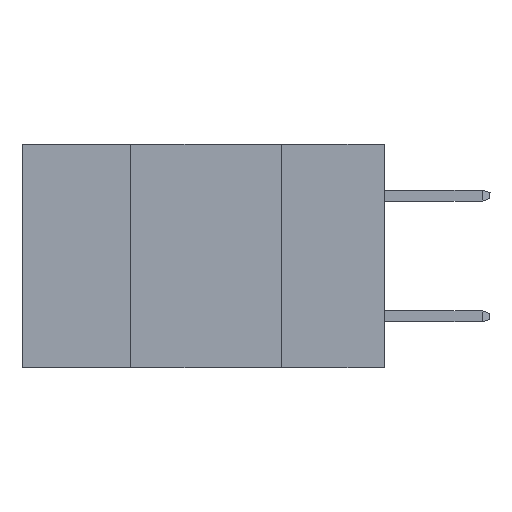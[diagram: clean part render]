
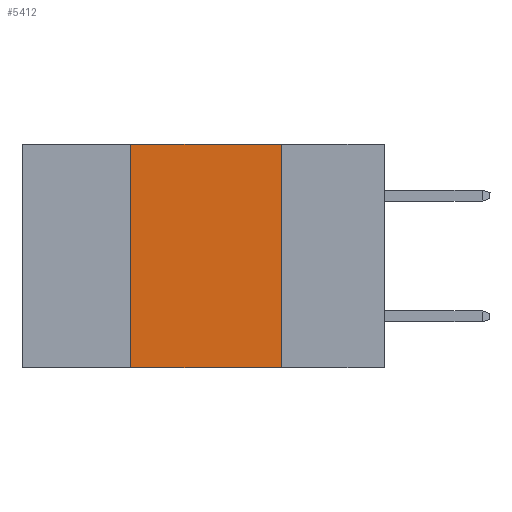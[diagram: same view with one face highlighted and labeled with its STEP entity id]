
A CAD part, left-side view. The second image highlights one B-rep face of the part: STEP entity #5412.
In plain terms, the highlighted planar face has unit normal (-1, 0, 0).
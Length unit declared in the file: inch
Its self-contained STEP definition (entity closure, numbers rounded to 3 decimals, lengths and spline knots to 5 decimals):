
#109 = PLANE ( 'NONE',  #27972 ) ;
#1936 = ORIENTED_EDGE ( 'NONE', *, *, #29631, .T. ) ;
#2480 = CARTESIAN_POINT ( 'NONE',  ( 0., 0.17, -0.37 ) ) ;
#3816 = EDGE_CURVE ( 'NONE', #24427, #20865, #25694, .T. ) ;
#4234 = VECTOR ( 'NONE', #25283, 39.37008 ) ;
#5412 = ADVANCED_FACE ( 'NONE', ( #25995 ), #109, .F. ) ;
#5451 = EDGE_LOOP ( 'NONE', ( #12696, #32093, #16387, #1936 ) ) ;
#5669 = CARTESIAN_POINT ( 'NONE',  ( 0., 0.6, 0. ) ) ;
#8476 = DIRECTION ( 'NONE',  ( 0., 0., -1. ) ) ;
#12034 = DIRECTION ( 'NONE',  ( 0., -1., 0. ) ) ;
#12310 = VECTOR ( 'NONE', #12034, 39.37008 ) ;
#12696 = ORIENTED_EDGE ( 'NONE', *, *, #13010, .F. ) ;
#13010 = EDGE_CURVE ( 'NONE', #31207, #27157, #28992, .T. ) ;
#13232 = CARTESIAN_POINT ( 'NONE',  ( 0., 0.17, 0. ) ) ;
#13496 = CARTESIAN_POINT ( 'NONE',  ( 0., 0.42, -0.37 ) ) ;
#15550 = CARTESIAN_POINT ( 'NONE',  ( 0., 0.6, -0.37 ) ) ;
#16387 = ORIENTED_EDGE ( 'NONE', *, *, #3816, .F. ) ;
#16401 = LINE ( 'NONE', #15550, #29676 ) ;
#18227 = CARTESIAN_POINT ( 'NONE',  ( 0., 0.42, 0. ) ) ;
#20865 = VERTEX_POINT ( 'NONE', #23949 ) ;
#21957 = VECTOR ( 'NONE', #29083, 39.37008 ) ;
#23949 = CARTESIAN_POINT ( 'NONE',  ( 0., 0.42, 0. ) ) ;
#24427 = VERTEX_POINT ( 'NONE', #13496 ) ;
#24458 = DIRECTION ( 'NONE',  ( 1., 0., 0. ) ) ;
#25283 = DIRECTION ( 'NONE',  ( 0., 0., 1. ) ) ;
#25407 = EDGE_CURVE ( 'NONE', #20865, #31207, #32517, .T. ) ;
#25694 = LINE ( 'NONE', #18227, #4234 ) ;
#25995 = FACE_OUTER_BOUND ( 'NONE', #5451, .T. ) ;
#27157 = VERTEX_POINT ( 'NONE', #2480 ) ;
#27902 = CARTESIAN_POINT ( 'NONE',  ( 0., 0.6, 0. ) ) ;
#27972 = AXIS2_PLACEMENT_3D ( 'NONE', #5669, #24458, #8476 ) ;
#28772 = DIRECTION ( 'NONE',  ( 0., -1., 0. ) ) ;
#28992 = LINE ( 'NONE', #13232, #21957 ) ;
#29083 = DIRECTION ( 'NONE',  ( 0., 0., -1. ) ) ;
#29631 = EDGE_CURVE ( 'NONE', #24427, #27157, #16401, .T. ) ;
#29676 = VECTOR ( 'NONE', #28772, 39.37008 ) ;
#31207 = VERTEX_POINT ( 'NONE', #32323 ) ;
#32093 = ORIENTED_EDGE ( 'NONE', *, *, #25407, .F. ) ;
#32323 = CARTESIAN_POINT ( 'NONE',  ( 0., 0.17, 0. ) ) ;
#32517 = LINE ( 'NONE', #27902, #12310 ) ;
